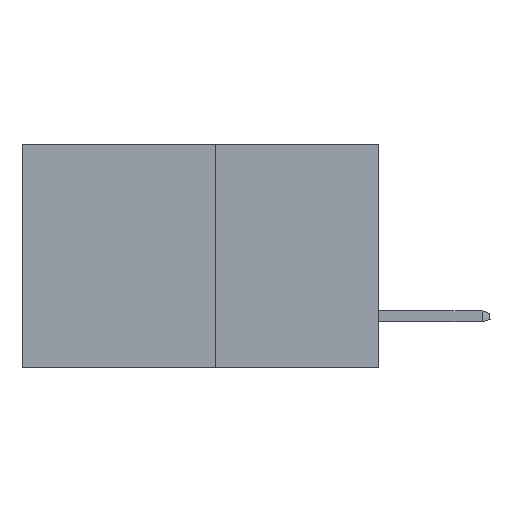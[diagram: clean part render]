
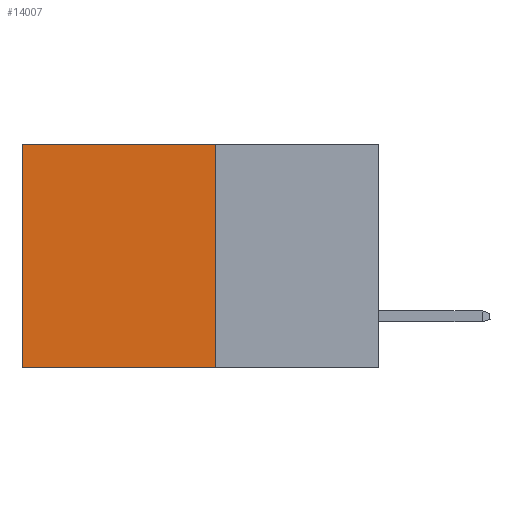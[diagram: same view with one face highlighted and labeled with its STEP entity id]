
A CAD part, left-side view. The second image highlights one B-rep face of the part: STEP entity #14007.
In plain terms, the highlighted planar face has unit normal (-1, 0, 0).
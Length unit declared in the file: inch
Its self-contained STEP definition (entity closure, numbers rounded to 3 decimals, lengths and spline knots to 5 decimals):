
#276 = EDGE_CURVE ( 'NONE', #9531, #9077, #3420, .T. ) ;
#902 = VERTEX_POINT ( 'NONE', #4200 ) ;
#2217 = DIRECTION ( 'NONE',  ( 0., 0., -1. ) ) ;
#2296 = ORIENTED_EDGE ( 'NONE', *, *, #2340, .T. ) ;
#2340 = EDGE_CURVE ( 'NONE', #6938, #902, #10451, .T. ) ;
#3202 = AXIS2_PLACEMENT_3D ( 'NONE', #15131, #14099, #7167 ) ;
#3264 = CARTESIAN_POINT ( 'NONE',  ( 0.277, 0.27, 0. ) ) ;
#3420 = LINE ( 'NONE', #8344, #6221 ) ;
#3582 = CARTESIAN_POINT ( 'NONE',  ( 0.277, 0.27, -0.37 ) ) ;
#4041 = DIRECTION ( 'NONE',  ( 0., 1., 0. ) ) ;
#4065 = ORIENTED_EDGE ( 'NONE', *, *, #276, .F. ) ;
#4200 = CARTESIAN_POINT ( 'NONE',  ( 0.277, 0.59, -0.37 ) ) ;
#4417 = ORIENTED_EDGE ( 'NONE', *, *, #13240, .T. ) ;
#5923 = PLANE ( 'NONE',  #3202 ) ;
#5941 = CARTESIAN_POINT ( 'NONE',  ( 0.277, 0.27, 0. ) ) ;
#6221 = VECTOR ( 'NONE', #12781, 39.37008 ) ;
#6444 = CARTESIAN_POINT ( 'NONE',  ( 0.277, 0.27, -0.37 ) ) ;
#6938 = VERTEX_POINT ( 'NONE', #11397 ) ;
#7167 = DIRECTION ( 'NONE',  ( 0., 0., -1. ) ) ;
#7469 = EDGE_CURVE ( 'NONE', #9077, #902, #11984, .T. ) ;
#8344 = CARTESIAN_POINT ( 'NONE',  ( 0.277, 0.27, -0.37 ) ) ;
#9077 = VERTEX_POINT ( 'NONE', #3582 ) ;
#9245 = VECTOR ( 'NONE', #4041, 39.37008 ) ;
#9271 = EDGE_LOOP ( 'NONE', ( #2296, #15512, #4065, #4417 ) ) ;
#9531 = VERTEX_POINT ( 'NONE', #3264 ) ;
#10092 = VECTOR ( 'NONE', #2217, 39.37008 ) ;
#10451 = LINE ( 'NONE', #11358, #10092 ) ;
#11358 = CARTESIAN_POINT ( 'NONE',  ( 0.277, 0.59, -0.37 ) ) ;
#11397 = CARTESIAN_POINT ( 'NONE',  ( 0.277, 0.59, 0. ) ) ;
#11559 = FACE_OUTER_BOUND ( 'NONE', #9271, .T. ) ;
#11915 = DIRECTION ( 'NONE',  ( 0., 1., 0. ) ) ;
#11939 = VECTOR ( 'NONE', #11915, 39.37008 ) ;
#11984 = LINE ( 'NONE', #6444, #9245 ) ;
#12781 = DIRECTION ( 'NONE',  ( 0., 0., -1. ) ) ;
#13240 = EDGE_CURVE ( 'NONE', #9531, #6938, #13373, .T. ) ;
#13373 = LINE ( 'NONE', #5941, #11939 ) ;
#14007 = ADVANCED_FACE ( 'NONE', ( #11559 ), #5923, .F. ) ;
#14099 = DIRECTION ( 'NONE',  ( 1., 0., 0. ) ) ;
#15131 = CARTESIAN_POINT ( 'NONE',  ( 0.277, 0.27, -0.37 ) ) ;
#15512 = ORIENTED_EDGE ( 'NONE', *, *, #7469, .F. ) ;
